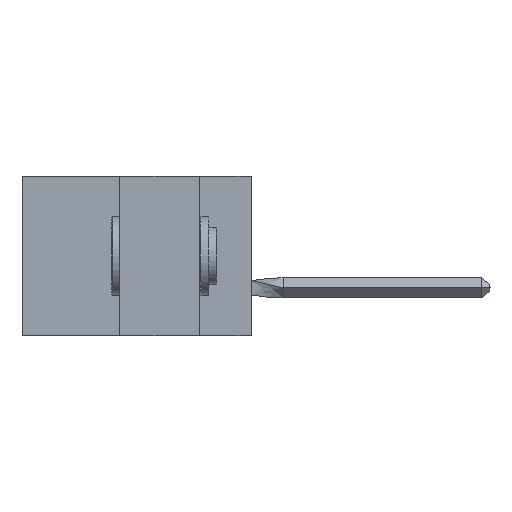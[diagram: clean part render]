
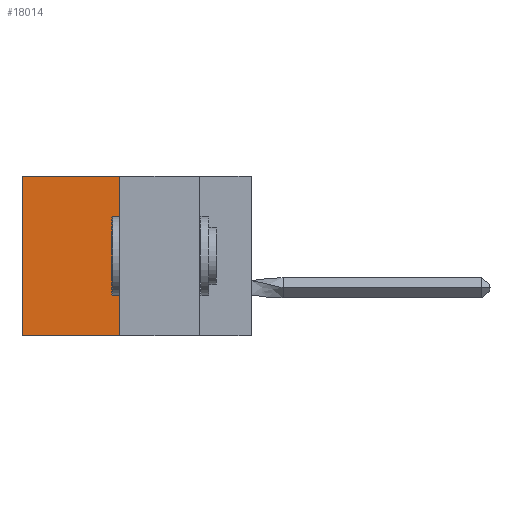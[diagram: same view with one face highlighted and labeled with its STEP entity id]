
A CAD part, left-side view. The second image highlights one B-rep face of the part: STEP entity #18014.
In plain terms, the highlighted planar face has unit normal (-1, 0, 0).
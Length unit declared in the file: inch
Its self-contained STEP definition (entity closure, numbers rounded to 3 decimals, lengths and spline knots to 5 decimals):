
#989 = VERTEX_POINT ( 'NONE', #3974 ) ;
#3974 = CARTESIAN_POINT ( 'NONE',  ( 0.305, 0.413, -0.5 ) ) ;
#4074 = AXIS2_PLACEMENT_3D ( 'NONE', #20804, #23734, #11399 ) ;
#4743 = VECTOR ( 'NONE', #27595, 39.37008 ) ;
#5223 = LINE ( 'NONE', #38087, #37490 ) ;
#5849 = VERTEX_POINT ( 'NONE', #13503 ) ;
#7973 = VERTEX_POINT ( 'NONE', #8552 ) ;
#8552 = CARTESIAN_POINT ( 'NONE',  ( 0.305, 0.72, -0.5 ) ) ;
#9399 = DIRECTION ( 'NONE',  ( 0., 1., 0. ) ) ;
#10232 = CARTESIAN_POINT ( 'NONE',  ( 0.305, 0.72, -0.5 ) ) ;
#11399 = DIRECTION ( 'NONE',  ( 0., 0., -1. ) ) ;
#13503 = CARTESIAN_POINT ( 'NONE',  ( 0.305, 0.72, 0. ) ) ;
#13860 = VECTOR ( 'NONE', #38380, 39.37008 ) ;
#14961 = CARTESIAN_POINT ( 'NONE',  ( 0.305, 0.413, -0.5 ) ) ;
#15059 = VECTOR ( 'NONE', #37445, 39.37008 ) ;
#18014 = ADVANCED_FACE ( 'NONE', ( #34599 ), #23608, .F. ) ;
#18786 = EDGE_CURVE ( 'NONE', #23846, #5849, #5223, .T. ) ;
#20804 = CARTESIAN_POINT ( 'NONE',  ( 0.305, 0.413, -0.5 ) ) ;
#21627 = LINE ( 'NONE', #24863, #4743 ) ;
#21863 = EDGE_CURVE ( 'NONE', #5849, #7973, #39666, .T. ) ;
#23524 = LINE ( 'NONE', #14961, #15059 ) ;
#23608 = PLANE ( 'NONE',  #4074 ) ;
#23726 = ORIENTED_EDGE ( 'NONE', *, *, #29978, .F. ) ;
#23734 = DIRECTION ( 'NONE',  ( 1., 0., 0. ) ) ;
#23846 = VERTEX_POINT ( 'NONE', #29788 ) ;
#24428 = ORIENTED_EDGE ( 'NONE', *, *, #26564, .F. ) ;
#24863 = CARTESIAN_POINT ( 'NONE',  ( 0.305, 0.413, -0.5 ) ) ;
#26564 = EDGE_CURVE ( 'NONE', #989, #7973, #23524, .T. ) ;
#27595 = DIRECTION ( 'NONE',  ( 0., 0., -1. ) ) ;
#29364 = ORIENTED_EDGE ( 'NONE', *, *, #21863, .T. ) ;
#29788 = CARTESIAN_POINT ( 'NONE',  ( 0.305, 0.413, 0. ) ) ;
#29978 = EDGE_CURVE ( 'NONE', #23846, #989, #21627, .T. ) ;
#34599 = FACE_OUTER_BOUND ( 'NONE', #38118, .T. ) ;
#37445 = DIRECTION ( 'NONE',  ( 0., 1., 0. ) ) ;
#37490 = VECTOR ( 'NONE', #9399, 39.37008 ) ;
#38087 = CARTESIAN_POINT ( 'NONE',  ( 0.305, 0.413, 0. ) ) ;
#38118 = EDGE_LOOP ( 'NONE', ( #29364, #24428, #23726, #38971 ) ) ;
#38380 = DIRECTION ( 'NONE',  ( 0., 0., -1. ) ) ;
#38971 = ORIENTED_EDGE ( 'NONE', *, *, #18786, .T. ) ;
#39666 = LINE ( 'NONE', #10232, #13860 ) ;
